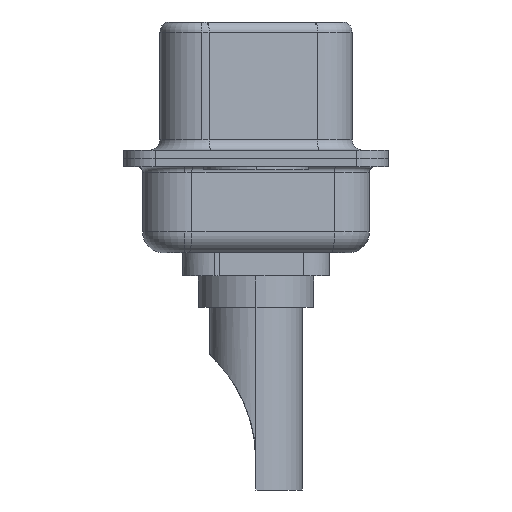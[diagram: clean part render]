
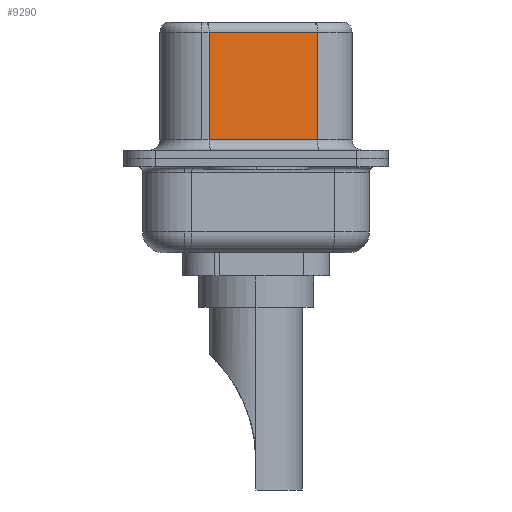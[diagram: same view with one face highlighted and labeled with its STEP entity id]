
A CAD part, left-side view. The second image highlights one B-rep face of the part: STEP entity #9290.
In plain terms, the highlighted planar face has unit normal (-0.985, -0.174, 0).
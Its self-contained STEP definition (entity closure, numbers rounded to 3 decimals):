
#261 = FACE_OUTER_BOUND ( 'NONE', #10511, .T. ) ;
#332 = CARTESIAN_POINT ( 'NONE',  ( 4.58, -2.927, 6.02 ) ) ;
#521 = CARTESIAN_POINT ( 'NONE',  ( 4.58, -2.927, 6.52 ) ) ;
#1477 = ORIENTED_EDGE ( 'NONE', *, *, #6411, .T. ) ;
#1524 = LINE ( 'NONE', #13739, #18878 ) ;
#2399 = ORIENTED_EDGE ( 'NONE', *, *, #3584, .T. ) ;
#2553 = VERTEX_POINT ( 'NONE', #17249 ) ;
#3584 = EDGE_CURVE ( 'NONE', #8882, #18269, #1524, .T. ) ;
#4008 = DIRECTION ( 'NONE',  ( -0.174, 0.985, 0. ) ) ;
#4474 = CARTESIAN_POINT ( 'NONE',  ( 3.67, 2.233, 0.9 ) ) ;
#4726 = EDGE_CURVE ( 'NONE', #8589, #18269, #15470, .T. ) ;
#4915 = DIRECTION ( 'NONE',  ( 0., 0., -1. ) ) ;
#5142 = VECTOR ( 'NONE', #4915, 1000. ) ;
#5999 = EDGE_CURVE ( 'NONE', #8589, #2553, #15981, .T. ) ;
#6411 = EDGE_CURVE ( 'NONE', #2553, #8882, #9673, .T. ) ;
#8589 = VERTEX_POINT ( 'NONE', #332 ) ;
#8882 = VERTEX_POINT ( 'NONE', #4474 ) ;
#9056 = CARTESIAN_POINT ( 'NONE',  ( 4.58, -2.927, 0.9 ) ) ;
#9290 = ADVANCED_FACE ( 'NONE', ( #261 ), #10747, .F. ) ;
#9673 = LINE ( 'NONE', #14347, #5142 ) ;
#10343 = AXIS2_PLACEMENT_3D ( 'NONE', #521, #14100, #4008 ) ;
#10511 = EDGE_LOOP ( 'NONE', ( #15846, #15570, #1477, #2399 ) ) ;
#10747 = PLANE ( 'NONE',  #10343 ) ;
#11259 = DIRECTION ( 'NONE',  ( 0.174, -0.985, 0. ) ) ;
#12733 = CARTESIAN_POINT ( 'NONE',  ( 4.58, -2.927, 6.52 ) ) ;
#13739 = CARTESIAN_POINT ( 'NONE',  ( 4.58, -2.927, 0.9 ) ) ;
#13966 = DIRECTION ( 'NONE',  ( -0.174, 0.985, 0. ) ) ;
#14100 = DIRECTION ( 'NONE',  ( 0.985, 0.174, 0. ) ) ;
#14347 = CARTESIAN_POINT ( 'NONE',  ( 3.67, 2.233, 6.52 ) ) ;
#15470 = LINE ( 'NONE', #12733, #20398 ) ;
#15570 = ORIENTED_EDGE ( 'NONE', *, *, #5999, .T. ) ;
#15846 = ORIENTED_EDGE ( 'NONE', *, *, #4726, .F. ) ;
#15981 = LINE ( 'NONE', #19121, #16505 ) ;
#16505 = VECTOR ( 'NONE', #13966, 1000. ) ;
#17249 = CARTESIAN_POINT ( 'NONE',  ( 3.67, 2.233, 6.02 ) ) ;
#18269 = VERTEX_POINT ( 'NONE', #9056 ) ;
#18878 = VECTOR ( 'NONE', #11259, 1000. ) ;
#19121 = CARTESIAN_POINT ( 'NONE',  ( 4.58, -2.927, 6.02 ) ) ;
#20298 = DIRECTION ( 'NONE',  ( 0., 0., -1. ) ) ;
#20398 = VECTOR ( 'NONE', #20298, 1000. ) ;
